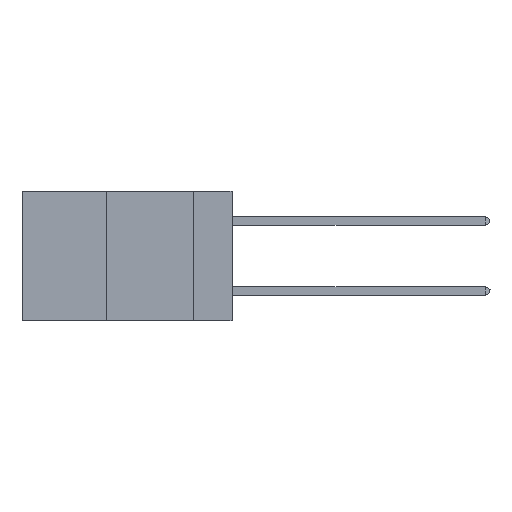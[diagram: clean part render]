
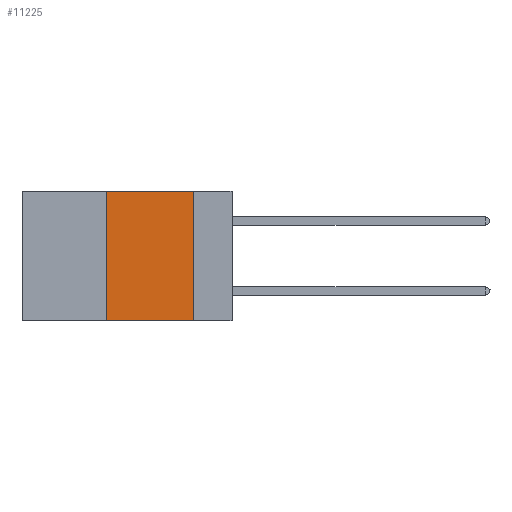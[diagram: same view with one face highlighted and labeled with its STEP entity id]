
A CAD part, left-side view. The second image highlights one B-rep face of the part: STEP entity #11225.
In plain terms, the highlighted planar face has unit normal (-1, 0, 0).
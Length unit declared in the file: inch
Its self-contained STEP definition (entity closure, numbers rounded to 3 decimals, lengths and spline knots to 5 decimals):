
#2909 = CARTESIAN_POINT ( 'NONE',  ( 0., 0.6, 0. ) ) ;
#3221 = ORIENTED_EDGE ( 'NONE', *, *, #17400, .F. ) ;
#4455 = ORIENTED_EDGE ( 'NONE', *, *, #20837, .F. ) ;
#5287 = EDGE_CURVE ( 'NONE', #28080, #16435, #9252, .T. ) ;
#5325 = CARTESIAN_POINT ( 'NONE',  ( 0., 0.36, 0. ) ) ;
#6386 = ORIENTED_EDGE ( 'NONE', *, *, #28601, .T. ) ;
#6675 = EDGE_LOOP ( 'NONE', ( #21107, #3221, #4455, #6386 ) ) ;
#6911 = CARTESIAN_POINT ( 'NONE',  ( 0., 0.11, 0. ) ) ;
#7610 = DIRECTION ( 'NONE',  ( 0., 0., 1. ) ) ;
#8078 = LINE ( 'NONE', #24727, #12934 ) ;
#9252 = LINE ( 'NONE', #6911, #19072 ) ;
#9438 = VECTOR ( 'NONE', #23399, 39.37008 ) ;
#10477 = CARTESIAN_POINT ( 'NONE',  ( 0., 0.11, -0.37 ) ) ;
#11225 = ADVANCED_FACE ( 'NONE', ( #12259 ), #29942, .F. ) ;
#11260 = AXIS2_PLACEMENT_3D ( 'NONE', #2909, #26725, #12722 ) ;
#11740 = DIRECTION ( 'NONE',  ( 0., 0., -1. ) ) ;
#12259 = FACE_OUTER_BOUND ( 'NONE', #6675, .T. ) ;
#12722 = DIRECTION ( 'NONE',  ( 0., 0., -1. ) ) ;
#12934 = VECTOR ( 'NONE', #17398, 39.37008 ) ;
#14045 = LINE ( 'NONE', #25561, #9438 ) ;
#14758 = LINE ( 'NONE', #21928, #18970 ) ;
#16435 = VERTEX_POINT ( 'NONE', #10477 ) ;
#17187 = VERTEX_POINT ( 'NONE', #28321 ) ;
#17398 = DIRECTION ( 'NONE',  ( 0., -1., 0. ) ) ;
#17400 = EDGE_CURVE ( 'NONE', #18097, #28080, #8078, .T. ) ;
#18097 = VERTEX_POINT ( 'NONE', #5325 ) ;
#18970 = VECTOR ( 'NONE', #7610, 39.37008 ) ;
#19072 = VECTOR ( 'NONE', #11740, 39.37008 ) ;
#19739 = CARTESIAN_POINT ( 'NONE',  ( 0., 0.11, 0. ) ) ;
#20837 = EDGE_CURVE ( 'NONE', #17187, #18097, #14758, .T. ) ;
#21107 = ORIENTED_EDGE ( 'NONE', *, *, #5287, .F. ) ;
#21928 = CARTESIAN_POINT ( 'NONE',  ( 0., 0.36, 0. ) ) ;
#23399 = DIRECTION ( 'NONE',  ( 0., -1., 0. ) ) ;
#24727 = CARTESIAN_POINT ( 'NONE',  ( 0., 0.6, 0. ) ) ;
#25561 = CARTESIAN_POINT ( 'NONE',  ( 0., 0.6, -0.37 ) ) ;
#26725 = DIRECTION ( 'NONE',  ( 1., 0., 0. ) ) ;
#28080 = VERTEX_POINT ( 'NONE', #19739 ) ;
#28321 = CARTESIAN_POINT ( 'NONE',  ( 0., 0.36, -0.37 ) ) ;
#28601 = EDGE_CURVE ( 'NONE', #17187, #16435, #14045, .T. ) ;
#29942 = PLANE ( 'NONE',  #11260 ) ;
